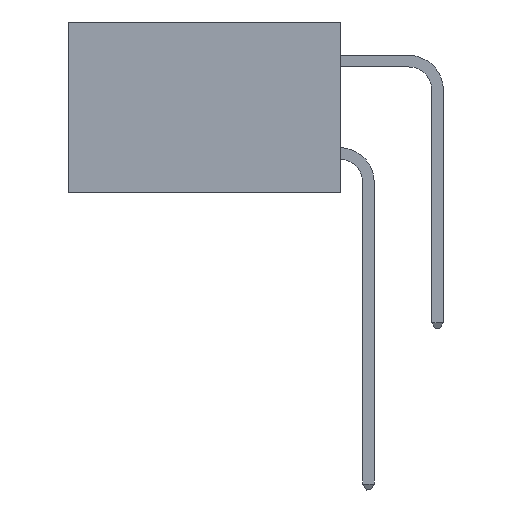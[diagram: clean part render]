
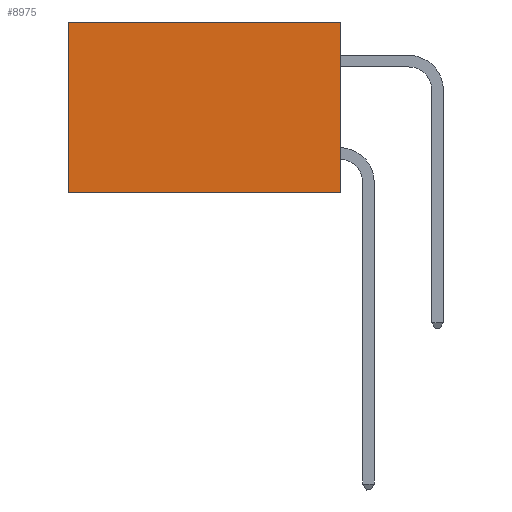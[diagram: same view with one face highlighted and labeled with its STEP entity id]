
A CAD part, left-side view. The second image highlights one B-rep face of the part: STEP entity #8975.
In plain terms, the highlighted planar face has unit normal (-1, 0, 0).
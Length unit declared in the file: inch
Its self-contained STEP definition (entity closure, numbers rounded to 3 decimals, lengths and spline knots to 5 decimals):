
#1441 = ORIENTED_EDGE ( 'NONE', *, *, #19068, .T. ) ;
#1789 = EDGE_CURVE ( 'NONE', #12649, #18115, #14642, .T. ) ;
#3635 = EDGE_LOOP ( 'NONE', ( #21586, #12585, #8597, #1441 ) ) ;
#4055 = CARTESIAN_POINT ( 'NONE',  ( 0.277, 0.59, 0. ) ) ;
#4152 = DIRECTION ( 'NONE',  ( 0., 0., -1. ) ) ;
#4227 = CARTESIAN_POINT ( 'NONE',  ( 0.277, 0., -0.37 ) ) ;
#4529 = CARTESIAN_POINT ( 'NONE',  ( 0.277, 0., 0. ) ) ;
#4670 = VECTOR ( 'NONE', #13682, 39.37008 ) ;
#5579 = VECTOR ( 'NONE', #7310, 39.37008 ) ;
#6760 = EDGE_CURVE ( 'NONE', #11350, #12649, #12779, .T. ) ;
#6922 = CARTESIAN_POINT ( 'NONE',  ( 0.277, 0., -0.37 ) ) ;
#7292 = CARTESIAN_POINT ( 'NONE',  ( 0.277, 0.59, -0.37 ) ) ;
#7310 = DIRECTION ( 'NONE',  ( 0., 0., -1. ) ) ;
#8597 = ORIENTED_EDGE ( 'NONE', *, *, #6760, .F. ) ;
#8629 = VERTEX_POINT ( 'NONE', #4055 ) ;
#8791 = DIRECTION ( 'NONE',  ( 0., 0., -1. ) ) ;
#8975 = ADVANCED_FACE ( 'NONE', ( #12400 ), #10596, .F. ) ;
#10596 = PLANE ( 'NONE',  #11129 ) ;
#11129 = AXIS2_PLACEMENT_3D ( 'NONE', #6922, #20094, #8791 ) ;
#11350 = VERTEX_POINT ( 'NONE', #17998 ) ;
#12065 = CARTESIAN_POINT ( 'NONE',  ( 0.277, 0., -0.37 ) ) ;
#12400 = FACE_OUTER_BOUND ( 'NONE', #3635, .T. ) ;
#12585 = ORIENTED_EDGE ( 'NONE', *, *, #1789, .F. ) ;
#12649 = VERTEX_POINT ( 'NONE', #12065 ) ;
#12779 = LINE ( 'NONE', #4227, #22205 ) ;
#12961 = CARTESIAN_POINT ( 'NONE',  ( 0.277, 0.59, -0.37 ) ) ;
#13682 = DIRECTION ( 'NONE',  ( 0., 1., 0. ) ) ;
#13825 = VECTOR ( 'NONE', #21460, 39.37008 ) ;
#14397 = EDGE_CURVE ( 'NONE', #8629, #18115, #20011, .T. ) ;
#14642 = LINE ( 'NONE', #19888, #4670 ) ;
#17998 = CARTESIAN_POINT ( 'NONE',  ( 0.277, 0., 0. ) ) ;
#18115 = VERTEX_POINT ( 'NONE', #7292 ) ;
#19068 = EDGE_CURVE ( 'NONE', #11350, #8629, #23811, .T. ) ;
#19888 = CARTESIAN_POINT ( 'NONE',  ( 0.277, 0., -0.37 ) ) ;
#20011 = LINE ( 'NONE', #12961, #5579 ) ;
#20094 = DIRECTION ( 'NONE',  ( 1., 0., 0. ) ) ;
#21460 = DIRECTION ( 'NONE',  ( 0., 1., 0. ) ) ;
#21586 = ORIENTED_EDGE ( 'NONE', *, *, #14397, .T. ) ;
#22205 = VECTOR ( 'NONE', #4152, 39.37008 ) ;
#23811 = LINE ( 'NONE', #4529, #13825 ) ;
